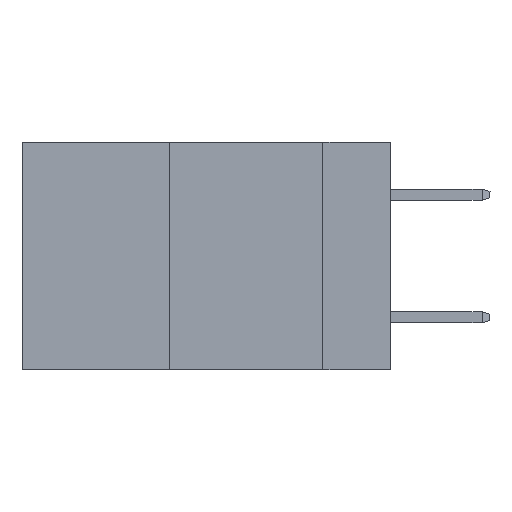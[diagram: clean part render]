
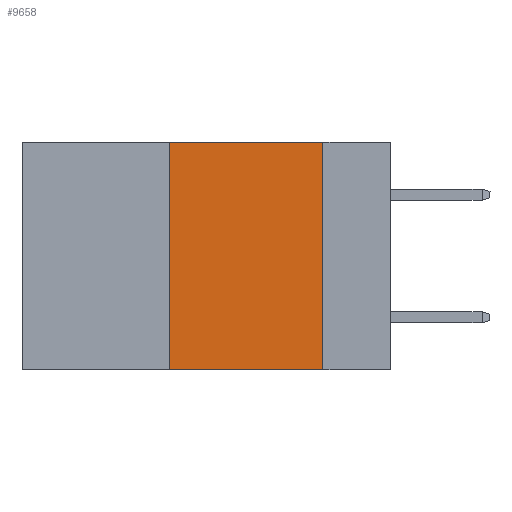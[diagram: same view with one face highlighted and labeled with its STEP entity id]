
A CAD part, left-side view. The second image highlights one B-rep face of the part: STEP entity #9658.
In plain terms, the highlighted planar face has unit normal (-1, 0, 0).
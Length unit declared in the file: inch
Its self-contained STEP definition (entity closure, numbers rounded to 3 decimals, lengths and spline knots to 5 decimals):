
#118 = CARTESIAN_POINT ( 'NONE',  ( 0., 0.36, 0. ) ) ;
#1192 = VECTOR ( 'NONE', #2178, 39.37008 ) ;
#1334 = CARTESIAN_POINT ( 'NONE',  ( 0., 0.36, -0.37 ) ) ;
#1386 = DIRECTION ( 'NONE',  ( 0., 0., -1. ) ) ;
#2178 = DIRECTION ( 'NONE',  ( 0., -1., 0. ) ) ;
#2731 = LINE ( 'NONE', #2864, #7829 ) ;
#2864 = CARTESIAN_POINT ( 'NONE',  ( 0., 0.36, 0. ) ) ;
#3323 = EDGE_CURVE ( 'NONE', #5811, #10261, #8107, .T. ) ;
#3809 = FACE_OUTER_BOUND ( 'NONE', #5865, .T. ) ;
#4511 = VERTEX_POINT ( 'NONE', #11026 ) ;
#4820 = VECTOR ( 'NONE', #1386, 39.37008 ) ;
#5361 = DIRECTION ( 'NONE',  ( 1., 0., 0. ) ) ;
#5523 = CARTESIAN_POINT ( 'NONE',  ( 0., 0.6, -0.37 ) ) ;
#5550 = DIRECTION ( 'NONE',  ( 0., 0., 1. ) ) ;
#5811 = VERTEX_POINT ( 'NONE', #118 ) ;
#5865 = EDGE_LOOP ( 'NONE', ( #10329, #5868, #10874, #7282 ) ) ;
#5868 = ORIENTED_EDGE ( 'NONE', *, *, #3323, .F. ) ;
#6436 = DIRECTION ( 'NONE',  ( 0., -1., 0. ) ) ;
#6677 = CARTESIAN_POINT ( 'NONE',  ( 0., 0.6, 0. ) ) ;
#6797 = CARTESIAN_POINT ( 'NONE',  ( 0., 0.11, 0. ) ) ;
#6967 = LINE ( 'NONE', #6797, #4820 ) ;
#7282 = ORIENTED_EDGE ( 'NONE', *, *, #8214, .T. ) ;
#7829 = VECTOR ( 'NONE', #5550, 39.37008 ) ;
#7981 = VECTOR ( 'NONE', #6436, 39.37008 ) ;
#8047 = PLANE ( 'NONE',  #9737 ) ;
#8107 = LINE ( 'NONE', #6677, #1192 ) ;
#8214 = EDGE_CURVE ( 'NONE', #10032, #4511, #10330, .T. ) ;
#8797 = EDGE_CURVE ( 'NONE', #10032, #5811, #2731, .T. ) ;
#9408 = EDGE_CURVE ( 'NONE', #10261, #4511, #6967, .T. ) ;
#9658 = ADVANCED_FACE ( 'NONE', ( #3809 ), #8047, .F. ) ;
#9737 = AXIS2_PLACEMENT_3D ( 'NONE', #9792, #5361, #11549 ) ;
#9792 = CARTESIAN_POINT ( 'NONE',  ( 0., 0.6, 0. ) ) ;
#10032 = VERTEX_POINT ( 'NONE', #1334 ) ;
#10261 = VERTEX_POINT ( 'NONE', #11468 ) ;
#10329 = ORIENTED_EDGE ( 'NONE', *, *, #9408, .F. ) ;
#10330 = LINE ( 'NONE', #5523, #7981 ) ;
#10874 = ORIENTED_EDGE ( 'NONE', *, *, #8797, .F. ) ;
#11026 = CARTESIAN_POINT ( 'NONE',  ( 0., 0.11, -0.37 ) ) ;
#11468 = CARTESIAN_POINT ( 'NONE',  ( 0., 0.11, 0. ) ) ;
#11549 = DIRECTION ( 'NONE',  ( 0., 0., -1. ) ) ;
